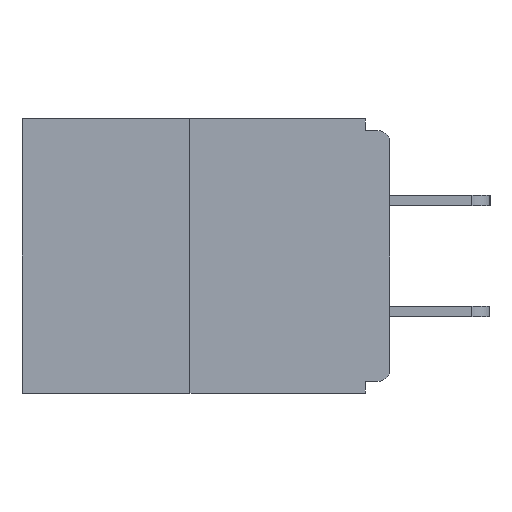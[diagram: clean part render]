
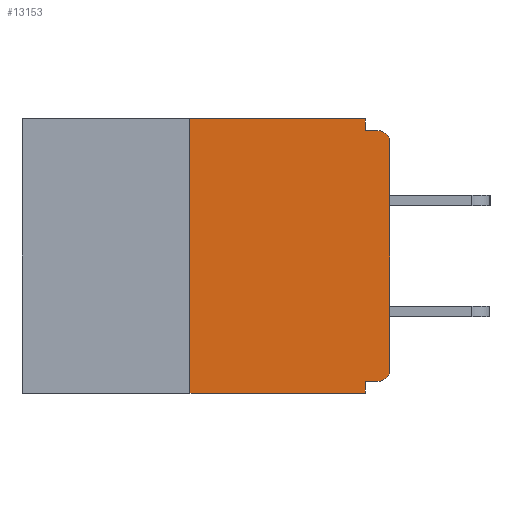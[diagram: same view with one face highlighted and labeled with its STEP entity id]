
A CAD part, left-side view. The second image highlights one B-rep face of the part: STEP entity #13153.
In plain terms, the highlighted planar face has unit normal (-1, 0, 0).
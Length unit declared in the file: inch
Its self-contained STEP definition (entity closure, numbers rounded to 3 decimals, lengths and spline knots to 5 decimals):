
#138 = EDGE_CURVE ( 'NONE', #20656, #545, #20143, .T. ) ;
#524 = DIRECTION ( 'NONE',  ( 1., 0., 0. ) ) ;
#542 = DIRECTION ( 'NONE',  ( 0., 0., -1. ) ) ;
#545 = VERTEX_POINT ( 'NONE', #18505 ) ;
#780 = CIRCLE ( 'NONE', #11763, 0.015 ) ;
#1168 = AXIS2_PLACEMENT_3D ( 'NONE', #17969, #524, #14639 ) ;
#1449 = VECTOR ( 'NONE', #4488, 39.37008 ) ;
#2061 = VERTEX_POINT ( 'NONE', #10202 ) ;
#2257 = CARTESIAN_POINT ( 'NONE',  ( 0., 0.031, -0.343 ) ) ;
#3730 = CARTESIAN_POINT ( 'NONE',  ( 0., 0.015, -0.313 ) ) ;
#3955 = VERTEX_POINT ( 'NONE', #12730 ) ;
#4418 = LINE ( 'NONE', #15104, #7387 ) ;
#4488 = DIRECTION ( 'NONE',  ( 0., 1., 0. ) ) ;
#4591 = VERTEX_POINT ( 'NONE', #22000 ) ;
#5272 = CARTESIAN_POINT ( 'NONE',  ( 0., 0.46, 0. ) ) ;
#5540 = CARTESIAN_POINT ( 'NONE',  ( 0., 0.015, -0.03 ) ) ;
#5615 = DIRECTION ( 'NONE',  ( 0., -1., 0. ) ) ;
#5673 = FACE_OUTER_BOUND ( 'NONE', #6064, .T. ) ;
#6064 = EDGE_LOOP ( 'NONE', ( #18249, #9860, #13446, #19276, #9215, #12568, #15222, #20447, #7909, #20029 ) ) ;
#6182 = CIRCLE ( 'NONE', #21984, 0.015 ) ;
#6284 = VECTOR ( 'NONE', #5615, 39.37008 ) ;
#6750 = VERTEX_POINT ( 'NONE', #17925 ) ;
#7152 = EDGE_CURVE ( 'NONE', #4591, #13775, #18014, .T. ) ;
#7365 = DIRECTION ( 'NONE',  ( 0., 0., -1. ) ) ;
#7387 = VECTOR ( 'NONE', #11773, 39.37008 ) ;
#7556 = EDGE_CURVE ( 'NONE', #2061, #545, #6182, .T. ) ;
#7909 = ORIENTED_EDGE ( 'NONE', *, *, #138, .F. ) ;
#8106 = LINE ( 'NONE', #18680, #12800 ) ;
#8623 = LINE ( 'NONE', #22674, #17618 ) ;
#8646 = VERTEX_POINT ( 'NONE', #16841 ) ;
#9215 = ORIENTED_EDGE ( 'NONE', *, *, #10989, .F. ) ;
#9860 = ORIENTED_EDGE ( 'NONE', *, *, #15849, .F. ) ;
#10059 = LINE ( 'NONE', #22481, #18080 ) ;
#10202 = CARTESIAN_POINT ( 'NONE',  ( 0., 0., -0.03 ) ) ;
#10744 = VERTEX_POINT ( 'NONE', #17840 ) ;
#10756 = DIRECTION ( 'NONE',  ( -1., 0., 0. ) ) ;
#10887 = DIRECTION ( 'NONE',  ( 0., 0., -1. ) ) ;
#10989 = EDGE_CURVE ( 'NONE', #6750, #4591, #22086, .T. ) ;
#11191 = DIRECTION ( 'NONE',  ( 0., -1., 0. ) ) ;
#11421 = CARTESIAN_POINT ( 'NONE',  ( 0., 0.031, -0.015 ) ) ;
#11763 = AXIS2_PLACEMENT_3D ( 'NONE', #3730, #10756, #542 ) ;
#11773 = DIRECTION ( 'NONE',  ( 0., 0., -1. ) ) ;
#12157 = EDGE_CURVE ( 'NONE', #10744, #13775, #8623, .T. ) ;
#12568 = ORIENTED_EDGE ( 'NONE', *, *, #17767, .T. ) ;
#12679 = PLANE ( 'NONE',  #1168 ) ;
#12730 = CARTESIAN_POINT ( 'NONE',  ( 0., 0.031, 0. ) ) ;
#12800 = VECTOR ( 'NONE', #20649, 39.37008 ) ;
#13153 = ADVANCED_FACE ( 'NONE', ( #5673 ), #12679, .F. ) ;
#13446 = ORIENTED_EDGE ( 'NONE', *, *, #12157, .T. ) ;
#13599 = EDGE_CURVE ( 'NONE', #21321, #3955, #14118, .T. ) ;
#13775 = VERTEX_POINT ( 'NONE', #21717 ) ;
#14118 = LINE ( 'NONE', #5272, #6284 ) ;
#14271 = DIRECTION ( 'NONE',  ( -1., 0., 0. ) ) ;
#14436 = EDGE_CURVE ( 'NONE', #8646, #2061, #10059, .T. ) ;
#14578 = CARTESIAN_POINT ( 'NONE',  ( 0., 0.25, 0. ) ) ;
#14639 = DIRECTION ( 'NONE',  ( 0., 0., -1. ) ) ;
#15091 = CARTESIAN_POINT ( 'NONE',  ( 0., 0., -0.015 ) ) ;
#15104 = CARTESIAN_POINT ( 'NONE',  ( 0., 0.031, 0. ) ) ;
#15222 = ORIENTED_EDGE ( 'NONE', *, *, #14436, .T. ) ;
#15394 = CARTESIAN_POINT ( 'NONE',  ( 0., 0., -0.328 ) ) ;
#15849 = EDGE_CURVE ( 'NONE', #10744, #21321, #8106, .T. ) ;
#15855 = VECTOR ( 'NONE', #11191, 39.37008 ) ;
#16841 = CARTESIAN_POINT ( 'NONE',  ( 0., 0., -0.313 ) ) ;
#17067 = DIRECTION ( 'NONE',  ( 0., 0., 1. ) ) ;
#17618 = VECTOR ( 'NONE', #21049, 39.37008 ) ;
#17767 = EDGE_CURVE ( 'NONE', #6750, #8646, #780, .T. ) ;
#17840 = CARTESIAN_POINT ( 'NONE',  ( 0., 0.25, -0.343 ) ) ;
#17925 = CARTESIAN_POINT ( 'NONE',  ( 0., 0.015, -0.328 ) ) ;
#17969 = CARTESIAN_POINT ( 'NONE',  ( 0., 0.46, 0. ) ) ;
#18014 = LINE ( 'NONE', #2257, #19384 ) ;
#18080 = VECTOR ( 'NONE', #17067, 39.37008 ) ;
#18249 = ORIENTED_EDGE ( 'NONE', *, *, #13599, .F. ) ;
#18505 = CARTESIAN_POINT ( 'NONE',  ( 0., 0.015, -0.015 ) ) ;
#18680 = CARTESIAN_POINT ( 'NONE',  ( 0., 0.25, 0. ) ) ;
#19145 = EDGE_CURVE ( 'NONE', #3955, #20656, #4418, .T. ) ;
#19276 = ORIENTED_EDGE ( 'NONE', *, *, #7152, .F. ) ;
#19384 = VECTOR ( 'NONE', #10887, 39.37008 ) ;
#20029 = ORIENTED_EDGE ( 'NONE', *, *, #19145, .F. ) ;
#20143 = LINE ( 'NONE', #15091, #15855 ) ;
#20447 = ORIENTED_EDGE ( 'NONE', *, *, #7556, .T. ) ;
#20649 = DIRECTION ( 'NONE',  ( 0., 0., 1. ) ) ;
#20656 = VERTEX_POINT ( 'NONE', #11421 ) ;
#21049 = DIRECTION ( 'NONE',  ( 0., -1., 0. ) ) ;
#21321 = VERTEX_POINT ( 'NONE', #14578 ) ;
#21717 = CARTESIAN_POINT ( 'NONE',  ( 0., 0.031, -0.343 ) ) ;
#21984 = AXIS2_PLACEMENT_3D ( 'NONE', #5540, #14271, #7365 ) ;
#22000 = CARTESIAN_POINT ( 'NONE',  ( 0., 0.031, -0.328 ) ) ;
#22086 = LINE ( 'NONE', #15394, #1449 ) ;
#22481 = CARTESIAN_POINT ( 'NONE',  ( 0., 0., 0. ) ) ;
#22674 = CARTESIAN_POINT ( 'NONE',  ( 0., 0.46, -0.343 ) ) ;
